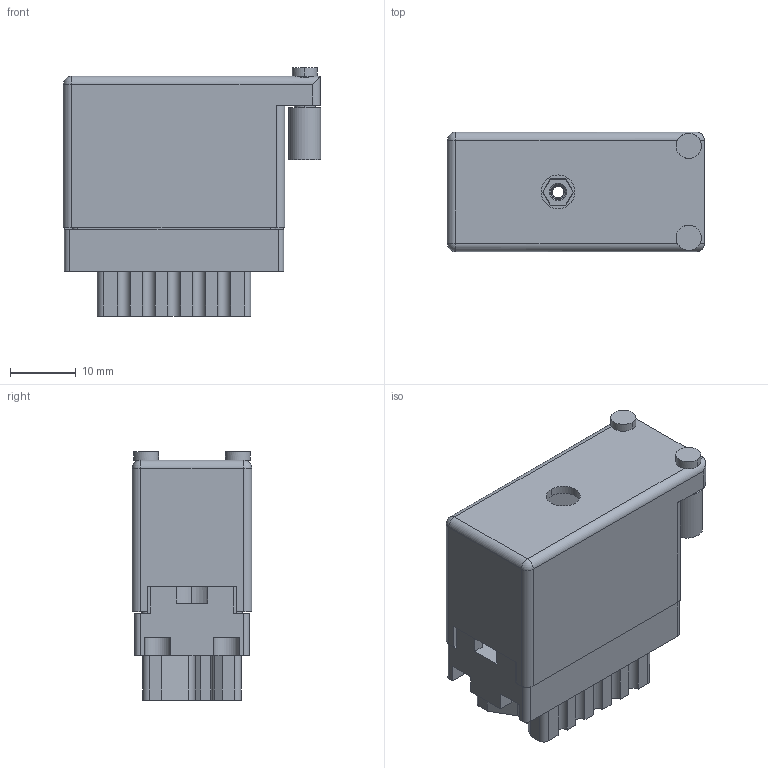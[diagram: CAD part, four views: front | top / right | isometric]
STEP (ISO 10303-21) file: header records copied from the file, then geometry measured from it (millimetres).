
FILE_DESCRIPTION (( 'STEP AP203' ), '1' );
FILE_NAME ('516-020-501-456.STEP', '2020-09-08T13:58:05', ( '' ), ( '' ), 'SwSTEP 2.0', 'SolidWorks 2020', '' );
FILE_SCHEMA (( 'CONFIG_CONTROL_DESIGN' ));
Length unit declared in the file: inch
Products named in the file (5): 516 Part Receptacle_020; 516-230-001_Metal - 020 Side Entry; 516-252-025-100_516-252-025-100; 516-020-501-456; 516-292-001_501 Contact
Assembly tree (23 placements, depth 2):
  516-020-501-456
    516 Part Receptacle_020
    516-292-001_501 Contact  x20
    516-230-001_Metal - 020 Side Entry
    516-252-025-100_516-252-025-100
Bounding box: 39.12 x 18.16 x 37.77 mm (x, y, z)
Volume: 9713.5 mm3; surface area: 18060.3 mm2
Topology: 23 solids, 23 shells, 2171 faces, 6278 edges, 4161 vertices
Faces by surface type: plane 1279, cylinder 756, bspline 123, cone 11, sphere 2
Entity records: 30444 total; most frequent: CARTESIAN_POINT 7730, ORIENTED_EDGE 4648, DIRECTION 4471, EDGE_CURVE 2324, LINE 1627, VECTOR 1627, VERTEX_POINT 1539, AXIS2_PLACEMENT_3D 1422
